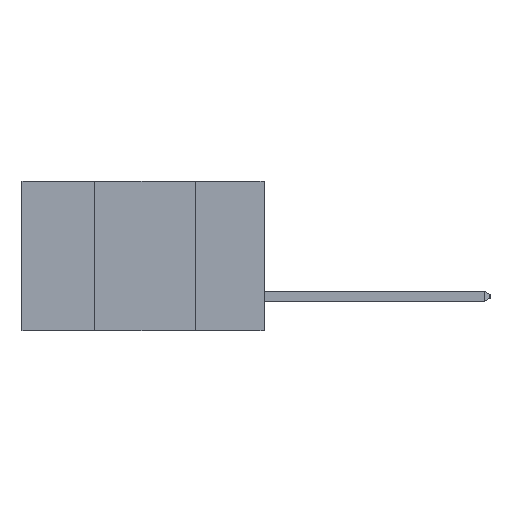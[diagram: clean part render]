
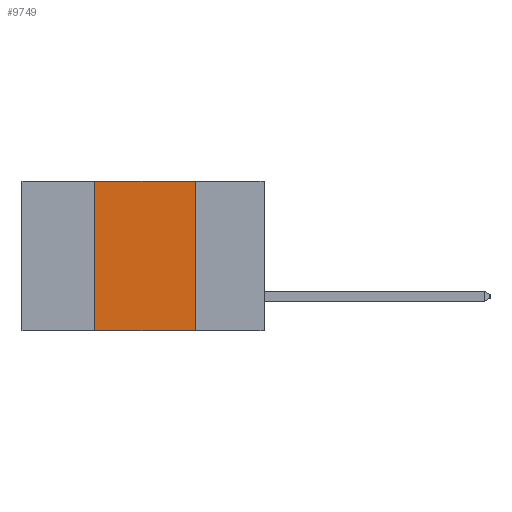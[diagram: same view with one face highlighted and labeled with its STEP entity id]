
A CAD part, left-side view. The second image highlights one B-rep face of the part: STEP entity #9749.
In plain terms, the highlighted planar face has unit normal (-1, 0, 0).
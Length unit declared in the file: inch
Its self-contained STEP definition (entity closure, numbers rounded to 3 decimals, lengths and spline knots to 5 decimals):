
#1189 = EDGE_CURVE ( 'NONE', #15383, #7826, #1741, .T. ) ;
#1251 = ORIENTED_EDGE ( 'NONE', *, *, #1189, .F. ) ;
#1741 = LINE ( 'NONE', #1815, #14436 ) ;
#1815 = CARTESIAN_POINT ( 'NONE',  ( 0., 0.6, 0. ) ) ;
#1946 = VECTOR ( 'NONE', #12968, 39.37008 ) ;
#1985 = ORIENTED_EDGE ( 'NONE', *, *, #14376, .F. ) ;
#2009 = CARTESIAN_POINT ( 'NONE',  ( 0., 0.6, 0. ) ) ;
#2394 = VERTEX_POINT ( 'NONE', #7338 ) ;
#2453 = EDGE_LOOP ( 'NONE', ( #1985, #1251, #3825, #6038 ) ) ;
#3317 = CARTESIAN_POINT ( 'NONE',  ( 0., 0.6, -0.37 ) ) ;
#3753 = DIRECTION ( 'NONE',  ( 0., 0., 1. ) ) ;
#3825 = ORIENTED_EDGE ( 'NONE', *, *, #13578, .F. ) ;
#4507 = CARTESIAN_POINT ( 'NONE',  ( 0., 0.17, 0. ) ) ;
#5220 = CARTESIAN_POINT ( 'NONE',  ( 0., 0.42, 0. ) ) ;
#5927 = DIRECTION ( 'NONE',  ( 0., 0., -1. ) ) ;
#6038 = ORIENTED_EDGE ( 'NONE', *, *, #10438, .T. ) ;
#6997 = CARTESIAN_POINT ( 'NONE',  ( 0., 0.17, 0. ) ) ;
#7338 = CARTESIAN_POINT ( 'NONE',  ( 0., 0.42, -0.37 ) ) ;
#7826 = VERTEX_POINT ( 'NONE', #6997 ) ;
#8077 = DIRECTION ( 'NONE',  ( 0., -1., 0. ) ) ;
#8962 = CARTESIAN_POINT ( 'NONE',  ( 0., 0.17, -0.37 ) ) ;
#9749 = ADVANCED_FACE ( 'NONE', ( #14198 ), #11918, .F. ) ;
#10123 = VECTOR ( 'NONE', #13082, 39.37008 ) ;
#10438 = EDGE_CURVE ( 'NONE', #2394, #13017, #13218, .T. ) ;
#11126 = CARTESIAN_POINT ( 'NONE',  ( 0., 0.42, 0. ) ) ;
#11834 = LINE ( 'NONE', #4507, #1946 ) ;
#11918 = PLANE ( 'NONE',  #12394 ) ;
#12385 = VECTOR ( 'NONE', #3753, 39.37008 ) ;
#12394 = AXIS2_PLACEMENT_3D ( 'NONE', #2009, #13102, #5927 ) ;
#12968 = DIRECTION ( 'NONE',  ( 0., 0., -1. ) ) ;
#13017 = VERTEX_POINT ( 'NONE', #8962 ) ;
#13082 = DIRECTION ( 'NONE',  ( 0., -1., 0. ) ) ;
#13102 = DIRECTION ( 'NONE',  ( 1., 0., 0. ) ) ;
#13218 = LINE ( 'NONE', #3317, #10123 ) ;
#13578 = EDGE_CURVE ( 'NONE', #2394, #15383, #15951, .T. ) ;
#14198 = FACE_OUTER_BOUND ( 'NONE', #2453, .T. ) ;
#14376 = EDGE_CURVE ( 'NONE', #7826, #13017, #11834, .T. ) ;
#14436 = VECTOR ( 'NONE', #8077, 39.37008 ) ;
#15383 = VERTEX_POINT ( 'NONE', #5220 ) ;
#15951 = LINE ( 'NONE', #11126, #12385 ) ;
